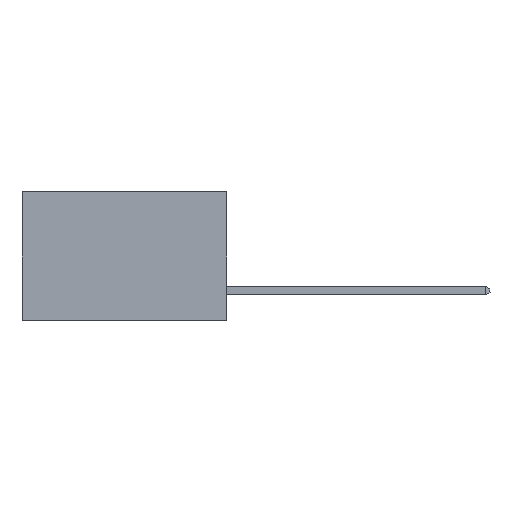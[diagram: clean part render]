
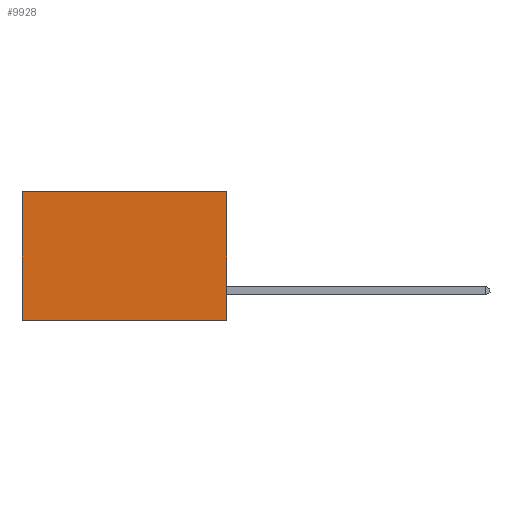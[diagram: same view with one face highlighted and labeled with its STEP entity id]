
A CAD part, left-side view. The second image highlights one B-rep face of the part: STEP entity #9928.
In plain terms, the highlighted planar face has unit normal (-1, 0, 0).
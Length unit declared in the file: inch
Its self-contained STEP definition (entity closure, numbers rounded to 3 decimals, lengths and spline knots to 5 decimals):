
#127 = CARTESIAN_POINT ( 'NONE',  ( 0.277, 0., 0. ) ) ;
#1798 = FACE_OUTER_BOUND ( 'NONE', #7107, .T. ) ;
#2621 = CARTESIAN_POINT ( 'NONE',  ( 0.277, 0., -0.37 ) ) ;
#2768 = DIRECTION ( 'NONE',  ( 0., 0., -1. ) ) ;
#2833 = DIRECTION ( 'NONE',  ( 0., 0., -1. ) ) ;
#2867 = DIRECTION ( 'NONE',  ( 1., 0., 0. ) ) ;
#2873 = PLANE ( 'NONE',  #4040 ) ;
#2948 = EDGE_CURVE ( 'NONE', #6766, #4951, #3406, .T. ) ;
#2990 = CARTESIAN_POINT ( 'NONE',  ( 0.277, 0., -0.37 ) ) ;
#3072 = CARTESIAN_POINT ( 'NONE',  ( 0.277, 0., -0.37 ) ) ;
#3212 = DIRECTION ( 'NONE',  ( 0., 1., 0. ) ) ;
#3398 = ORIENTED_EDGE ( 'NONE', *, *, #13479, .T. ) ;
#3406 = LINE ( 'NONE', #2621, #13328 ) ;
#3623 = ORIENTED_EDGE ( 'NONE', *, *, #2948, .F. ) ;
#4040 = AXIS2_PLACEMENT_3D ( 'NONE', #2990, #2867, #2833 ) ;
#4902 = CARTESIAN_POINT ( 'NONE',  ( 0.277, 0.59, -0.37 ) ) ;
#4951 = VERTEX_POINT ( 'NONE', #8679 ) ;
#5106 = ORIENTED_EDGE ( 'NONE', *, *, #8496, .T. ) ;
#5660 = DIRECTION ( 'NONE',  ( 0., 1., 0. ) ) ;
#5683 = VERTEX_POINT ( 'NONE', #4902 ) ;
#6766 = VERTEX_POINT ( 'NONE', #9918 ) ;
#6830 = VERTEX_POINT ( 'NONE', #10649 ) ;
#7107 = EDGE_LOOP ( 'NONE', ( #5106, #7894, #3623, #3398 ) ) ;
#7302 = CARTESIAN_POINT ( 'NONE',  ( 0.277, 0.59, -0.37 ) ) ;
#7306 = DIRECTION ( 'NONE',  ( 0., 0., -1. ) ) ;
#7486 = LINE ( 'NONE', #7302, #8114 ) ;
#7880 = EDGE_CURVE ( 'NONE', #4951, #5683, #10786, .T. ) ;
#7894 = ORIENTED_EDGE ( 'NONE', *, *, #7880, .F. ) ;
#8114 = VECTOR ( 'NONE', #7306, 39.37008 ) ;
#8496 = EDGE_CURVE ( 'NONE', #6830, #5683, #7486, .T. ) ;
#8679 = CARTESIAN_POINT ( 'NONE',  ( 0.277, 0., -0.37 ) ) ;
#9918 = CARTESIAN_POINT ( 'NONE',  ( 0.277, 0., 0. ) ) ;
#9928 = ADVANCED_FACE ( 'NONE', ( #1798 ), #2873, .F. ) ;
#10121 = VECTOR ( 'NONE', #3212, 39.37008 ) ;
#10649 = CARTESIAN_POINT ( 'NONE',  ( 0.277, 0.59, 0. ) ) ;
#10786 = LINE ( 'NONE', #3072, #10121 ) ;
#12261 = VECTOR ( 'NONE', #5660, 39.37008 ) ;
#12573 = LINE ( 'NONE', #127, #12261 ) ;
#13328 = VECTOR ( 'NONE', #2768, 39.37008 ) ;
#13479 = EDGE_CURVE ( 'NONE', #6766, #6830, #12573, .T. ) ;
